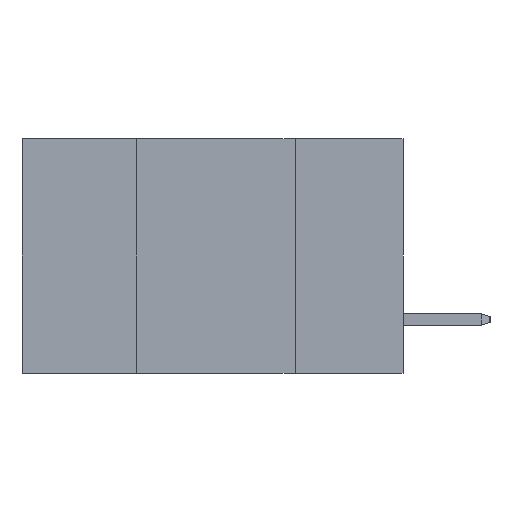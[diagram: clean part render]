
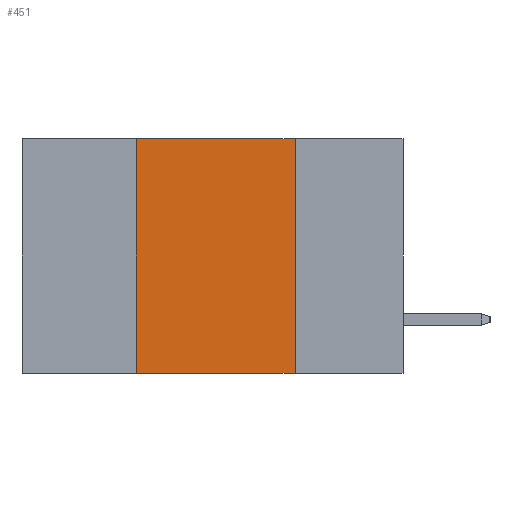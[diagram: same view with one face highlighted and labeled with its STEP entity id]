
A CAD part, left-side view. The second image highlights one B-rep face of the part: STEP entity #451.
In plain terms, the highlighted planar face has unit normal (-1, 0, 0).
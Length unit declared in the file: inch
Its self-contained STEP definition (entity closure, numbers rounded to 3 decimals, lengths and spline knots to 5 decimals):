
#15 = CARTESIAN_POINT ( 'NONE',  ( 0., 0.17, 0. ) ) ;
#334 = VECTOR ( 'NONE', #1830, 39.37008 ) ;
#423 = DIRECTION ( 'NONE',  ( 0., 0., 1. ) ) ;
#451 = ADVANCED_FACE ( 'NONE', ( #11764 ), #6307, .F. ) ;
#1229 = CARTESIAN_POINT ( 'NONE',  ( 0., 0.6, 0. ) ) ;
#1249 = ORIENTED_EDGE ( 'NONE', *, *, #11880, .F. ) ;
#1787 = VECTOR ( 'NONE', #5952, 39.37008 ) ;
#1830 = DIRECTION ( 'NONE',  ( 0., -1., 0. ) ) ;
#2069 = DIRECTION ( 'NONE',  ( 0., 0., -1. ) ) ;
#2181 = CARTESIAN_POINT ( 'NONE',  ( 0., 0.42, -0.37 ) ) ;
#2514 = VERTEX_POINT ( 'NONE', #15 ) ;
#2525 = ORIENTED_EDGE ( 'NONE', *, *, #7656, .F. ) ;
#2997 = EDGE_LOOP ( 'NONE', ( #10644, #1249, #2525, #3196 ) ) ;
#3196 = ORIENTED_EDGE ( 'NONE', *, *, #4853, .T. ) ;
#3456 = CARTESIAN_POINT ( 'NONE',  ( 0., 0.42, 0. ) ) ;
#4079 = VERTEX_POINT ( 'NONE', #12691 ) ;
#4729 = LINE ( 'NONE', #5781, #7687 ) ;
#4853 = EDGE_CURVE ( 'NONE', #10567, #4079, #8182, .T. ) ;
#4896 = CARTESIAN_POINT ( 'NONE',  ( 0., 0.6, -0.37 ) ) ;
#5013 = CARTESIAN_POINT ( 'NONE',  ( 0., 0.6, 0. ) ) ;
#5237 = LINE ( 'NONE', #9515, #10007 ) ;
#5781 = CARTESIAN_POINT ( 'NONE',  ( 0., 0.42, 0. ) ) ;
#5952 = DIRECTION ( 'NONE',  ( 0., -1., 0. ) ) ;
#6307 = PLANE ( 'NONE',  #7044 ) ;
#7044 = AXIS2_PLACEMENT_3D ( 'NONE', #1229, #9734, #12799 ) ;
#7656 = EDGE_CURVE ( 'NONE', #10567, #13281, #4729, .T. ) ;
#7687 = VECTOR ( 'NONE', #423, 39.37008 ) ;
#8182 = LINE ( 'NONE', #4896, #1787 ) ;
#9515 = CARTESIAN_POINT ( 'NONE',  ( 0., 0.17, 0. ) ) ;
#9734 = DIRECTION ( 'NONE',  ( 1., 0., 0. ) ) ;
#10007 = VECTOR ( 'NONE', #2069, 39.37008 ) ;
#10567 = VERTEX_POINT ( 'NONE', #2181 ) ;
#10644 = ORIENTED_EDGE ( 'NONE', *, *, #12810, .F. ) ;
#11764 = FACE_OUTER_BOUND ( 'NONE', #2997, .T. ) ;
#11880 = EDGE_CURVE ( 'NONE', #13281, #2514, #13477, .T. ) ;
#12691 = CARTESIAN_POINT ( 'NONE',  ( 0., 0.17, -0.37 ) ) ;
#12799 = DIRECTION ( 'NONE',  ( 0., 0., -1. ) ) ;
#12810 = EDGE_CURVE ( 'NONE', #2514, #4079, #5237, .T. ) ;
#13281 = VERTEX_POINT ( 'NONE', #3456 ) ;
#13477 = LINE ( 'NONE', #5013, #334 ) ;
